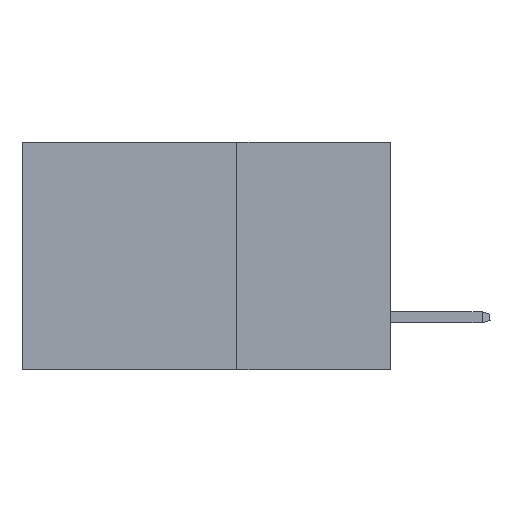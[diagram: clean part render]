
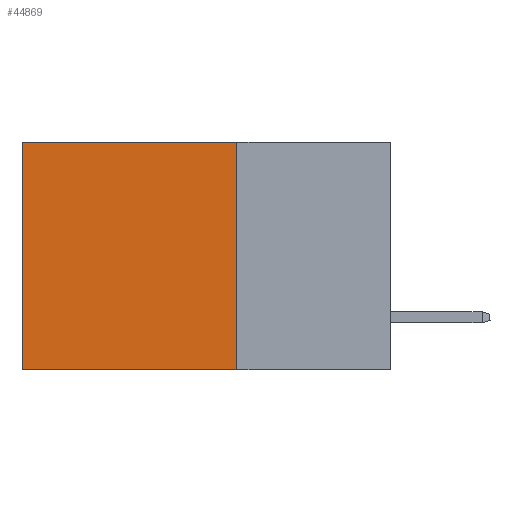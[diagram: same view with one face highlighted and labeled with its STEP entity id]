
A CAD part, left-side view. The second image highlights one B-rep face of the part: STEP entity #44869.
In plain terms, the highlighted planar face has unit normal (-1, 0, 0).
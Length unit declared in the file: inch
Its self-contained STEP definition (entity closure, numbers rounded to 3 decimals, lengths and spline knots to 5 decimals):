
#962 = VECTOR ( 'NONE', #10536, 39.37008 ) ;
#2781 = FACE_OUTER_BOUND ( 'NONE', #10868, .T. ) ;
#4765 = DIRECTION ( 'NONE',  ( 1., 0., 0. ) ) ;
#6552 = VERTEX_POINT ( 'NONE', #10502 ) ;
#8300 = CARTESIAN_POINT ( 'NONE',  ( 0.2875, 0.25, 0. ) ) ;
#9740 = LINE ( 'NONE', #18825, #22256 ) ;
#10502 = CARTESIAN_POINT ( 'NONE',  ( 0.2875, 0.6, -0.37 ) ) ;
#10536 = DIRECTION ( 'NONE',  ( 0., 1., 0. ) ) ;
#10868 = EDGE_LOOP ( 'NONE', ( #44852, #10989, #20668, #20301 ) ) ;
#10989 = ORIENTED_EDGE ( 'NONE', *, *, #13387, .F. ) ;
#12041 = CARTESIAN_POINT ( 'NONE',  ( 0.2875, 0.6, 0. ) ) ;
#12139 = VECTOR ( 'NONE', #43863, 39.37008 ) ;
#13387 = EDGE_CURVE ( 'NONE', #24708, #6552, #35927, .T. ) ;
#13421 = CARTESIAN_POINT ( 'NONE',  ( 0.2875, 0.25, -0.37 ) ) ;
#18825 = CARTESIAN_POINT ( 'NONE',  ( 0.2875, 0.25, 0. ) ) ;
#19510 = CARTESIAN_POINT ( 'NONE',  ( 0.2875, 0.25, 0. ) ) ;
#19632 = CARTESIAN_POINT ( 'NONE',  ( 0.2875, 0.6, 0. ) ) ;
#20006 = DIRECTION ( 'NONE',  ( 0., 0., -1. ) ) ;
#20301 = ORIENTED_EDGE ( 'NONE', *, *, #22091, .T. ) ;
#20668 = ORIENTED_EDGE ( 'NONE', *, *, #29767, .F. ) ;
#21104 = VERTEX_POINT ( 'NONE', #8300 ) ;
#22091 = EDGE_CURVE ( 'NONE', #21104, #33231, #32951, .T. ) ;
#22256 = VECTOR ( 'NONE', #45008, 39.37008 ) ;
#24708 = VERTEX_POINT ( 'NONE', #13421 ) ;
#28056 = VECTOR ( 'NONE', #20006, 39.37008 ) ;
#29767 = EDGE_CURVE ( 'NONE', #21104, #24708, #9740, .T. ) ;
#32951 = LINE ( 'NONE', #36230, #12139 ) ;
#33231 = VERTEX_POINT ( 'NONE', #19632 ) ;
#35577 = AXIS2_PLACEMENT_3D ( 'NONE', #19510, #4765, #46312 ) ;
#35927 = LINE ( 'NONE', #44183, #962 ) ;
#36230 = CARTESIAN_POINT ( 'NONE',  ( 0.2875, 0.25, 0. ) ) ;
#36364 = LINE ( 'NONE', #12041, #28056 ) ;
#42484 = PLANE ( 'NONE',  #35577 ) ;
#43863 = DIRECTION ( 'NONE',  ( 0., 1., 0. ) ) ;
#44183 = CARTESIAN_POINT ( 'NONE',  ( 0.2875, 0.25, -0.37 ) ) ;
#44852 = ORIENTED_EDGE ( 'NONE', *, *, #46745, .T. ) ;
#44869 = ADVANCED_FACE ( 'NONE', ( #2781 ), #42484, .F. ) ;
#45008 = DIRECTION ( 'NONE',  ( 0., 0., -1. ) ) ;
#46312 = DIRECTION ( 'NONE',  ( 0., 0., -1. ) ) ;
#46745 = EDGE_CURVE ( 'NONE', #33231, #6552, #36364, .T. ) ;
